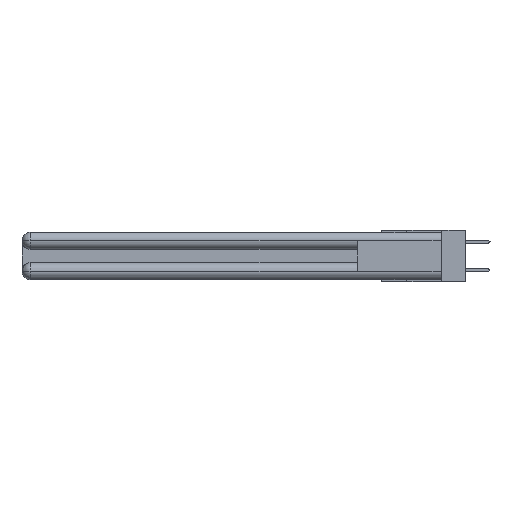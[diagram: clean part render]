
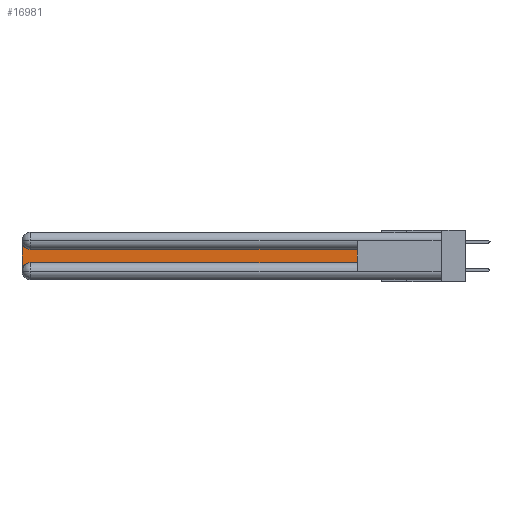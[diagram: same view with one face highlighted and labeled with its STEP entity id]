
A CAD part, left-side view. The second image highlights one B-rep face of the part: STEP entity #16981.
In plain terms, the highlighted planar face has unit normal (-1, 0, 0).
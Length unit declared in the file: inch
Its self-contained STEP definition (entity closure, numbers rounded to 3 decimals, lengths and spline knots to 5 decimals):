
#1679 = DIRECTION ( 'NONE',  ( 0., 0., -1. ) ) ;
#1794 = CARTESIAN_POINT ( 'NONE',  ( 0.075, 2.94, -0.2775 ) ) ;
#1959 = EDGE_CURVE ( 'NONE', #28604, #28713, #26334, .T. ) ;
#2352 = DIRECTION ( 'NONE',  ( 0., 0., 1. ) ) ;
#3358 = DIRECTION ( 'NONE',  ( 0., 0., -1. ) ) ;
#3946 = DIRECTION ( 'NONE',  ( 1., 0., 0. ) ) ;
#4390 = PLANE ( 'NONE',  #9927 ) ;
#5151 = CARTESIAN_POINT ( 'NONE',  ( 0.075, 2.94, -0.0625 ) ) ;
#5584 = FACE_OUTER_BOUND ( 'NONE', #17378, .T. ) ;
#5661 = CIRCLE ( 'NONE', #9310, 0.06 ) ;
#5750 = VERTEX_POINT ( 'NONE', #17954 ) ;
#6312 = EDGE_CURVE ( 'NONE', #5750, #28604, #31382, .T. ) ;
#6335 = VERTEX_POINT ( 'NONE', #22599 ) ;
#6820 = VERTEX_POINT ( 'NONE', #28489 ) ;
#7018 = CARTESIAN_POINT ( 'NONE',  ( 0.075, 3., -0.1225 ) ) ;
#7100 = EDGE_CURVE ( 'NONE', #6820, #5750, #16074, .T. ) ;
#7841 = CARTESIAN_POINT ( 'NONE',  ( 0.075, 0.6, -0.2175 ) ) ;
#8743 = VECTOR ( 'NONE', #3358, 39.37008 ) ;
#9310 = AXIS2_PLACEMENT_3D ( 'NONE', #5151, #20731, #26405 ) ;
#9401 = ORIENTED_EDGE ( 'NONE', *, *, #21011, .T. ) ;
#9585 = LINE ( 'NONE', #16464, #8743 ) ;
#9927 = AXIS2_PLACEMENT_3D ( 'NONE', #7018, #3946, #22530 ) ;
#11286 = EDGE_CURVE ( 'NONE', #18602, #6820, #9585, .T. ) ;
#11307 = DIRECTION ( 'NONE',  ( 0., 1., 0. ) ) ;
#11544 = EDGE_CURVE ( 'NONE', #28713, #6335, #30291, .T. ) ;
#11564 = VECTOR ( 'NONE', #30613, 39.37008 ) ;
#12317 = ORIENTED_EDGE ( 'NONE', *, *, #6312, .T. ) ;
#13063 = ORIENTED_EDGE ( 'NONE', *, *, #1959, .T. ) ;
#13086 = VECTOR ( 'NONE', #2352, 39.37008 ) ;
#16074 = CIRCLE ( 'NONE', #19218, 0.06 ) ;
#16464 = CARTESIAN_POINT ( 'NONE',  ( 0.075, 3., -0.2175 ) ) ;
#16981 = ADVANCED_FACE ( 'NONE', ( #5584 ), #4390, .F. ) ;
#17378 = EDGE_LOOP ( 'NONE', ( #33537, #9401, #20196, #28431, #12317, #13063 ) ) ;
#17954 = CARTESIAN_POINT ( 'NONE',  ( 0.075, 2.94, -0.2175 ) ) ;
#18602 = VERTEX_POINT ( 'NONE', #22996 ) ;
#19218 = AXIS2_PLACEMENT_3D ( 'NONE', #1794, #20471, #1679 ) ;
#19616 = CARTESIAN_POINT ( 'NONE',  ( 0.075, 0.6, -0.1225 ) ) ;
#20196 = ORIENTED_EDGE ( 'NONE', *, *, #11286, .T. ) ;
#20471 = DIRECTION ( 'NONE',  ( 1., 0., 0. ) ) ;
#20731 = DIRECTION ( 'NONE',  ( 1., 0., 0. ) ) ;
#21011 = EDGE_CURVE ( 'NONE', #6335, #18602, #5661, .T. ) ;
#22530 = DIRECTION ( 'NONE',  ( 0., 0., -1. ) ) ;
#22599 = CARTESIAN_POINT ( 'NONE',  ( 0.075, 2.94, -0.1225 ) ) ;
#22942 = CARTESIAN_POINT ( 'NONE',  ( 0.075, 0.6, -0.2175 ) ) ;
#22996 = CARTESIAN_POINT ( 'NONE',  ( 0.075, 3., -0.0625 ) ) ;
#26334 = LINE ( 'NONE', #7841, #13086 ) ;
#26405 = DIRECTION ( 'NONE',  ( 0., 0., -1. ) ) ;
#28431 = ORIENTED_EDGE ( 'NONE', *, *, #7100, .T. ) ;
#28489 = CARTESIAN_POINT ( 'NONE',  ( 0.075, 3., -0.2775 ) ) ;
#28604 = VERTEX_POINT ( 'NONE', #30146 ) ;
#28713 = VERTEX_POINT ( 'NONE', #30595 ) ;
#30146 = CARTESIAN_POINT ( 'NONE',  ( 0.075, 0.6, -0.2175 ) ) ;
#30291 = LINE ( 'NONE', #19616, #33580 ) ;
#30595 = CARTESIAN_POINT ( 'NONE',  ( 0.075, 0.6, -0.1225 ) ) ;
#30613 = DIRECTION ( 'NONE',  ( 0., -1., 0. ) ) ;
#31382 = LINE ( 'NONE', #22942, #11564 ) ;
#33537 = ORIENTED_EDGE ( 'NONE', *, *, #11544, .T. ) ;
#33580 = VECTOR ( 'NONE', #11307, 39.37008 ) ;
